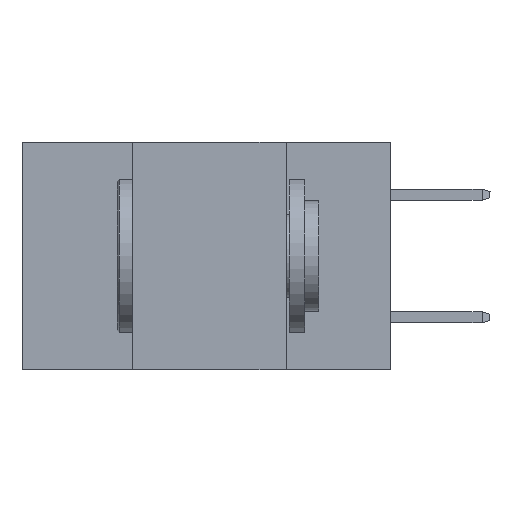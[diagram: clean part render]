
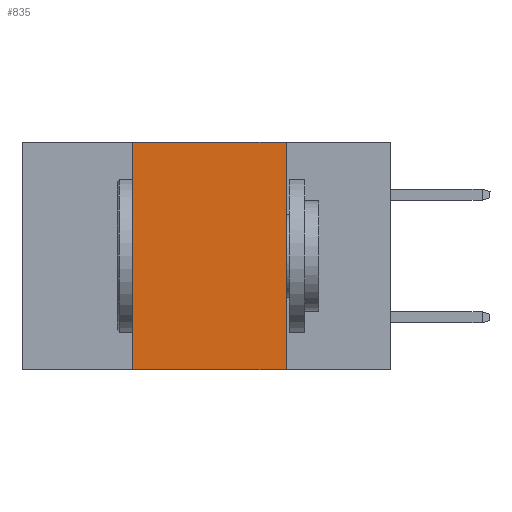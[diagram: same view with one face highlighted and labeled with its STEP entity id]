
A CAD part, left-side view. The second image highlights one B-rep face of the part: STEP entity #835.
In plain terms, the highlighted planar face has unit normal (-1, 0, 0).
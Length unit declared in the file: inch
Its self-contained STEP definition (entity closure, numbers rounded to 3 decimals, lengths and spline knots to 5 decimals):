
#37 = AXIS2_PLACEMENT_3D ( 'NONE', #5317, #5384, #7666 ) ;
#466 = ORIENTED_EDGE ( 'NONE', *, *, #2648, .F. ) ;
#609 = VERTEX_POINT ( 'NONE', #6329 ) ;
#835 = ADVANCED_FACE ( 'NONE', ( #7711 ), #8376, .F. ) ;
#1002 = CARTESIAN_POINT ( 'NONE',  ( 0., 0.42, 0. ) ) ;
#1295 = LINE ( 'NONE', #3845, #8708 ) ;
#1634 = VECTOR ( 'NONE', #2915, 39.37008 ) ;
#2049 = VERTEX_POINT ( 'NONE', #1002 ) ;
#2632 = VECTOR ( 'NONE', #9285, 39.37008 ) ;
#2648 = EDGE_CURVE ( 'NONE', #2049, #3790, #1295, .T. ) ;
#2686 = CARTESIAN_POINT ( 'NONE',  ( 0., 0.17, -0.37 ) ) ;
#2915 = DIRECTION ( 'NONE',  ( 0., 0., -1. ) ) ;
#3020 = DIRECTION ( 'NONE',  ( 0., -1., 0. ) ) ;
#3470 = EDGE_CURVE ( 'NONE', #3790, #8110, #7647, .T. ) ;
#3790 = VERTEX_POINT ( 'NONE', #7778 ) ;
#3845 = CARTESIAN_POINT ( 'NONE',  ( 0., 0.6, 0. ) ) ;
#4123 = VECTOR ( 'NONE', #6739, 39.37008 ) ;
#4270 = CARTESIAN_POINT ( 'NONE',  ( 0., 0.42, 0. ) ) ;
#4462 = ORIENTED_EDGE ( 'NONE', *, *, #9457, .T. ) ;
#5317 = CARTESIAN_POINT ( 'NONE',  ( 0., 0.6, 0. ) ) ;
#5384 = DIRECTION ( 'NONE',  ( 1., 0., 0. ) ) ;
#5745 = LINE ( 'NONE', #4270, #4123 ) ;
#5908 = ORIENTED_EDGE ( 'NONE', *, *, #3470, .F. ) ;
#6013 = EDGE_LOOP ( 'NONE', ( #5908, #466, #9744, #4462 ) ) ;
#6329 = CARTESIAN_POINT ( 'NONE',  ( 0., 0.42, -0.37 ) ) ;
#6562 = EDGE_CURVE ( 'NONE', #609, #2049, #5745, .T. ) ;
#6739 = DIRECTION ( 'NONE',  ( 0., 0., 1. ) ) ;
#7647 = LINE ( 'NONE', #8200, #1634 ) ;
#7666 = DIRECTION ( 'NONE',  ( 0., 0., -1. ) ) ;
#7711 = FACE_OUTER_BOUND ( 'NONE', #6013, .T. ) ;
#7778 = CARTESIAN_POINT ( 'NONE',  ( 0., 0.17, 0. ) ) ;
#8110 = VERTEX_POINT ( 'NONE', #2686 ) ;
#8200 = CARTESIAN_POINT ( 'NONE',  ( 0., 0.17, 0. ) ) ;
#8376 = PLANE ( 'NONE',  #37 ) ;
#8413 = LINE ( 'NONE', #8422, #2632 ) ;
#8422 = CARTESIAN_POINT ( 'NONE',  ( 0., 0.6, -0.37 ) ) ;
#8708 = VECTOR ( 'NONE', #3020, 39.37008 ) ;
#9285 = DIRECTION ( 'NONE',  ( 0., -1., 0. ) ) ;
#9457 = EDGE_CURVE ( 'NONE', #609, #8110, #8413, .T. ) ;
#9744 = ORIENTED_EDGE ( 'NONE', *, *, #6562, .F. ) ;
